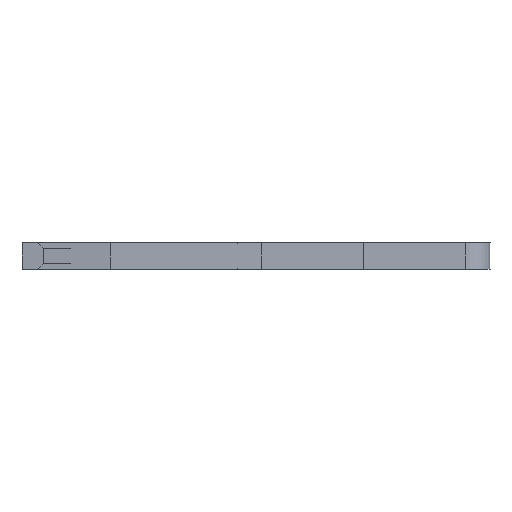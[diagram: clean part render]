
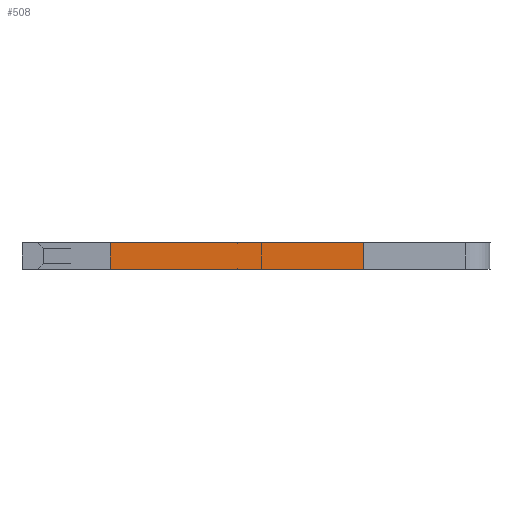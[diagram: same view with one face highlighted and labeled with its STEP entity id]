
A CAD part, left-side view. The second image highlights one B-rep face of the part: STEP entity #508.
In plain terms, the highlighted face is planar.
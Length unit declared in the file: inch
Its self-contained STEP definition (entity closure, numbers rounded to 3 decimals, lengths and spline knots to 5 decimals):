
#35 = DIRECTION ( 'NONE',  ( 1., 0., 0. ) ) ;
#46 = ORIENTED_EDGE ( 'NONE', *, *, #829, .F. ) ;
#112 = LINE ( 'NONE', #2721, #1769 ) ;
#146 = LINE ( 'NONE', #2673, #1122 ) ;
#283 = VERTEX_POINT ( 'NONE', #2006 ) ;
#447 = EDGE_CURVE ( 'NONE', #2165, #1992, #146, .T. ) ;
#508 = ADVANCED_FACE ( 'NONE', ( #2054 ), #1542, .F. ) ;
#554 = CARTESIAN_POINT ( 'NONE',  ( 0.013, 0.146, -0.0575 ) ) ;
#659 = LINE ( 'NONE', #554, #905 ) ;
#670 = VERTEX_POINT ( 'NONE', #1315 ) ;
#829 = EDGE_CURVE ( 'NONE', #670, #1992, #112, .T. ) ;
#905 = VECTOR ( 'NONE', #2743, 39.37008 ) ;
#1122 = VECTOR ( 'NONE', #1985, 39.37008 ) ;
#1124 = VECTOR ( 'NONE', #1611, 39.37008 ) ;
#1133 = LINE ( 'NONE', #2529, #1124 ) ;
#1177 = ORIENTED_EDGE ( 'NONE', *, *, #1491, .F. ) ;
#1287 = AXIS2_PLACEMENT_3D ( 'NONE', #1766, #2637, #35 ) ;
#1315 = CARTESIAN_POINT ( 'NONE',  ( 0.013, 0.146, -0.0575 ) ) ;
#1403 = DIRECTION ( 'NONE',  ( -1., 0., 0. ) ) ;
#1491 = EDGE_CURVE ( 'NONE', #283, #670, #659, .T. ) ;
#1535 = EDGE_CURVE ( 'NONE', #283, #2165, #1133, .T. ) ;
#1542 = PLANE ( 'NONE',  #1287 ) ;
#1611 = DIRECTION ( 'NONE',  ( -1., 0., 0. ) ) ;
#1737 = CARTESIAN_POINT ( 'NONE',  ( -0.013, -0.099, -0.0575 ) ) ;
#1766 = CARTESIAN_POINT ( 'NONE',  ( 0.013, 0.146, -0.0575 ) ) ;
#1769 = VECTOR ( 'NONE', #1403, 39.37008 ) ;
#1829 = EDGE_LOOP ( 'NONE', ( #2371, #46, #1177, #1921 ) ) ;
#1921 = ORIENTED_EDGE ( 'NONE', *, *, #1535, .T. ) ;
#1964 = CARTESIAN_POINT ( 'NONE',  ( -0.013, 0.146, -0.0575 ) ) ;
#1985 = DIRECTION ( 'NONE',  ( 0., 1., 0. ) ) ;
#1992 = VERTEX_POINT ( 'NONE', #1964 ) ;
#2006 = CARTESIAN_POINT ( 'NONE',  ( 0.013, -0.099, -0.0575 ) ) ;
#2054 = FACE_OUTER_BOUND ( 'NONE', #1829, .T. ) ;
#2165 = VERTEX_POINT ( 'NONE', #1737 ) ;
#2371 = ORIENTED_EDGE ( 'NONE', *, *, #447, .T. ) ;
#2529 = CARTESIAN_POINT ( 'NONE',  ( 0.013, -0.099, -0.0575 ) ) ;
#2637 = DIRECTION ( 'NONE',  ( 0., 0., 1. ) ) ;
#2673 = CARTESIAN_POINT ( 'NONE',  ( -0.013, 0.146, -0.0575 ) ) ;
#2721 = CARTESIAN_POINT ( 'NONE',  ( 0.013, 0.146, -0.0575 ) ) ;
#2743 = DIRECTION ( 'NONE',  ( 0., 1., 0. ) ) ;
